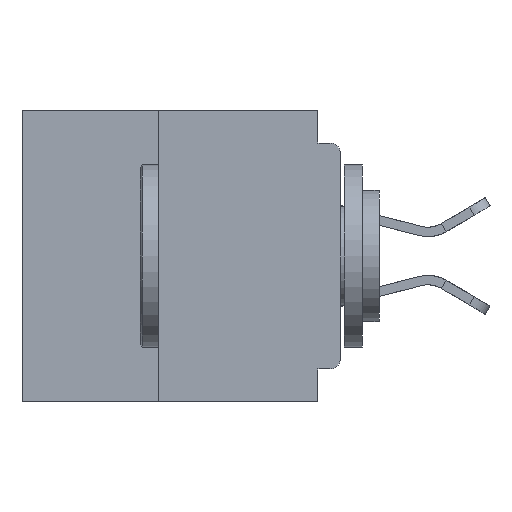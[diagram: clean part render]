
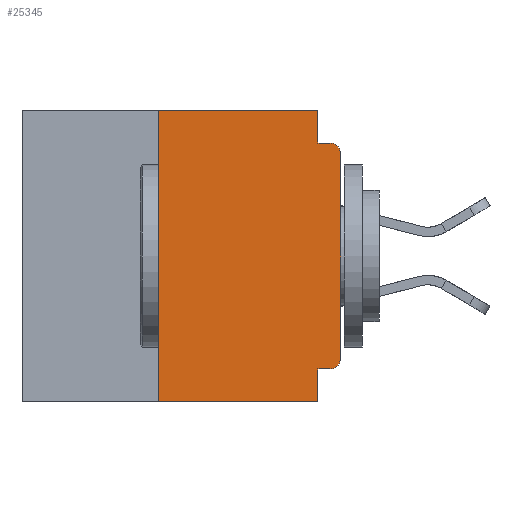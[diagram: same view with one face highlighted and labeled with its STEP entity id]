
A CAD part, left-side view. The second image highlights one B-rep face of the part: STEP entity #25345.
In plain terms, the highlighted planar face has unit normal (-1, 0, 0).
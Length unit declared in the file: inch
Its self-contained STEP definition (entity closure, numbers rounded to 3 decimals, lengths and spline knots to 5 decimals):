
#197 = CARTESIAN_POINT ( 'NONE',  ( 0., 0.015, -0.34 ) ) ;
#670 = CARTESIAN_POINT ( 'NONE',  ( 0., 0.437, -0.4 ) ) ;
#684 = VECTOR ( 'NONE', #27176, 39.37008 ) ;
#1099 = AXIS2_PLACEMENT_3D ( 'NONE', #29988, #14376, #36126 ) ;
#2647 = ORIENTED_EDGE ( 'NONE', *, *, #8266, .F. ) ;
#3069 = CARTESIAN_POINT ( 'NONE',  ( 0., 0.031, -0.4 ) ) ;
#3225 = CARTESIAN_POINT ( 'NONE',  ( 0., 0.031, 0. ) ) ;
#3390 = VERTEX_POINT ( 'NONE', #5452 ) ;
#3428 = DIRECTION ( 'NONE',  ( 0., 0., -1. ) ) ;
#3511 = CARTESIAN_POINT ( 'NONE',  ( 0., 0., -0.34 ) ) ;
#4297 = VERTEX_POINT ( 'NONE', #18903 ) ;
#5265 = CARTESIAN_POINT ( 'NONE',  ( 0., 0., 0. ) ) ;
#5313 = ORIENTED_EDGE ( 'NONE', *, *, #8869, .T. ) ;
#5452 = CARTESIAN_POINT ( 'NONE',  ( 0., 0.015, -0.045 ) ) ;
#5467 = EDGE_CURVE ( 'NONE', #31591, #33028, #17391, .T. ) ;
#6156 = CARTESIAN_POINT ( 'NONE',  ( 0., 0.015, -0.355 ) ) ;
#6608 = LINE ( 'NONE', #38926, #20277 ) ;
#7140 = LINE ( 'NONE', #3225, #14458 ) ;
#8104 = PLANE ( 'NONE',  #1099 ) ;
#8266 = EDGE_CURVE ( 'NONE', #39539, #31591, #35130, .T. ) ;
#8869 = EDGE_CURVE ( 'NONE', #39539, #21222, #13682, .T. ) ;
#8911 = CARTESIAN_POINT ( 'NONE',  ( 0., 0.031, -0.355 ) ) ;
#9714 = CARTESIAN_POINT ( 'NONE',  ( 0., 0.015, -0.06 ) ) ;
#10338 = VECTOR ( 'NONE', #15742, 39.37008 ) ;
#10860 = VERTEX_POINT ( 'NONE', #6156 ) ;
#11067 = DIRECTION ( 'NONE',  ( 0., -1., 0. ) ) ;
#11878 = LINE ( 'NONE', #37416, #20138 ) ;
#12341 = CARTESIAN_POINT ( 'NONE',  ( 0., 0.25, -0.4 ) ) ;
#12393 = VECTOR ( 'NONE', #17736, 39.37008 ) ;
#12861 = DIRECTION ( 'NONE',  ( 0., 0., -1. ) ) ;
#13682 = LINE ( 'NONE', #670, #29349 ) ;
#14376 = DIRECTION ( 'NONE',  ( 1., 0., 0. ) ) ;
#14458 = VECTOR ( 'NONE', #34397, 39.37008 ) ;
#14581 = CARTESIAN_POINT ( 'NONE',  ( 0., 0., -0.355 ) ) ;
#14766 = EDGE_CURVE ( 'NONE', #10860, #37811, #20233, .T. ) ;
#14911 = EDGE_CURVE ( 'NONE', #20515, #3390, #6608, .T. ) ;
#14972 = EDGE_LOOP ( 'NONE', ( #25762, #20086, #38252, #30968, #30421, #2647, #5313, #34545, #28067, #24469 ) ) ;
#15160 = DIRECTION ( 'NONE',  ( 0., -1., 0. ) ) ;
#15742 = DIRECTION ( 'NONE',  ( 0., 0., 1. ) ) ;
#15821 = CIRCLE ( 'NONE', #26462, 0.015 ) ;
#16410 = VECTOR ( 'NONE', #15160, 39.37008 ) ;
#17391 = LINE ( 'NONE', #24526, #16410 ) ;
#17736 = DIRECTION ( 'NONE',  ( 0., 1., 0. ) ) ;
#18798 = DIRECTION ( 'NONE',  ( 0., 0., -1. ) ) ;
#18903 = CARTESIAN_POINT ( 'NONE',  ( 0., 0., -0.06 ) ) ;
#19813 = EDGE_CURVE ( 'NONE', #37811, #4297, #34964, .T. ) ;
#20085 = EDGE_CURVE ( 'NONE', #4297, #3390, #15821, .T. ) ;
#20086 = ORIENTED_EDGE ( 'NONE', *, *, #20085, .T. ) ;
#20138 = VECTOR ( 'NONE', #18798, 39.37008 ) ;
#20233 = CIRCLE ( 'NONE', #34899, 0.015 ) ;
#20277 = VECTOR ( 'NONE', #11067, 39.37008 ) ;
#20515 = VERTEX_POINT ( 'NONE', #24204 ) ;
#21222 = VERTEX_POINT ( 'NONE', #3069 ) ;
#22224 = DIRECTION ( 'NONE',  ( -1., 0., 0. ) ) ;
#24204 = CARTESIAN_POINT ( 'NONE',  ( 0., 0.031, -0.045 ) ) ;
#24469 = ORIENTED_EDGE ( 'NONE', *, *, #14766, .T. ) ;
#24526 = CARTESIAN_POINT ( 'NONE',  ( 0., 0.437, 0. ) ) ;
#25137 = EDGE_CURVE ( 'NONE', #33028, #20515, #7140, .T. ) ;
#25345 = ADVANCED_FACE ( 'NONE', ( #39735 ), #8104, .F. ) ;
#25762 = ORIENTED_EDGE ( 'NONE', *, *, #19813, .T. ) ;
#26462 = AXIS2_PLACEMENT_3D ( 'NONE', #9714, #31515, #12861 ) ;
#27176 = DIRECTION ( 'NONE',  ( 0., 0., 1. ) ) ;
#28067 = ORIENTED_EDGE ( 'NONE', *, *, #36956, .F. ) ;
#28384 = VERTEX_POINT ( 'NONE', #8911 ) ;
#28733 = CARTESIAN_POINT ( 'NONE',  ( 0., 0.031, 0. ) ) ;
#29349 = VECTOR ( 'NONE', #38148, 39.37008 ) ;
#29988 = CARTESIAN_POINT ( 'NONE',  ( 0., 0.437, 0. ) ) ;
#30421 = ORIENTED_EDGE ( 'NONE', *, *, #5467, .F. ) ;
#30968 = ORIENTED_EDGE ( 'NONE', *, *, #25137, .F. ) ;
#31439 = CARTESIAN_POINT ( 'NONE',  ( 0., 0.25, -0.4 ) ) ;
#31515 = DIRECTION ( 'NONE',  ( -1., 0., 0. ) ) ;
#31591 = VERTEX_POINT ( 'NONE', #40152 ) ;
#33028 = VERTEX_POINT ( 'NONE', #28733 ) ;
#34397 = DIRECTION ( 'NONE',  ( 0., 0., -1. ) ) ;
#34545 = ORIENTED_EDGE ( 'NONE', *, *, #37177, .F. ) ;
#34899 = AXIS2_PLACEMENT_3D ( 'NONE', #197, #22224, #3428 ) ;
#34964 = LINE ( 'NONE', #5265, #684 ) ;
#35130 = LINE ( 'NONE', #31439, #10338 ) ;
#36126 = DIRECTION ( 'NONE',  ( 0., 0., -1. ) ) ;
#36956 = EDGE_CURVE ( 'NONE', #10860, #28384, #37164, .T. ) ;
#37164 = LINE ( 'NONE', #14581, #12393 ) ;
#37177 = EDGE_CURVE ( 'NONE', #28384, #21222, #11878, .T. ) ;
#37416 = CARTESIAN_POINT ( 'NONE',  ( 0., 0.031, -0.4 ) ) ;
#37811 = VERTEX_POINT ( 'NONE', #3511 ) ;
#38148 = DIRECTION ( 'NONE',  ( 0., -1., 0. ) ) ;
#38252 = ORIENTED_EDGE ( 'NONE', *, *, #14911, .F. ) ;
#38926 = CARTESIAN_POINT ( 'NONE',  ( 0., 0., -0.045 ) ) ;
#39539 = VERTEX_POINT ( 'NONE', #12341 ) ;
#39735 = FACE_OUTER_BOUND ( 'NONE', #14972, .T. ) ;
#40152 = CARTESIAN_POINT ( 'NONE',  ( 0., 0.25, 0. ) ) ;
